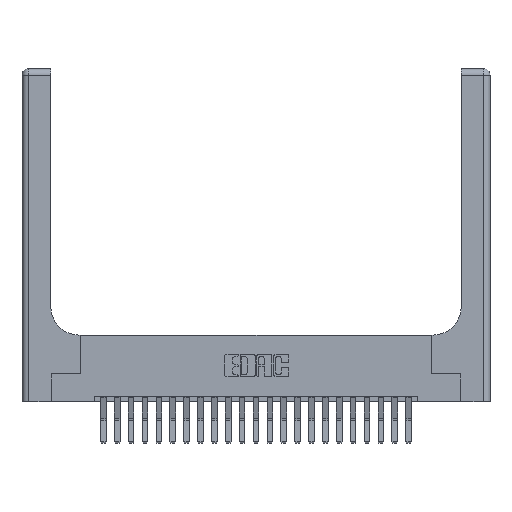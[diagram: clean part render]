
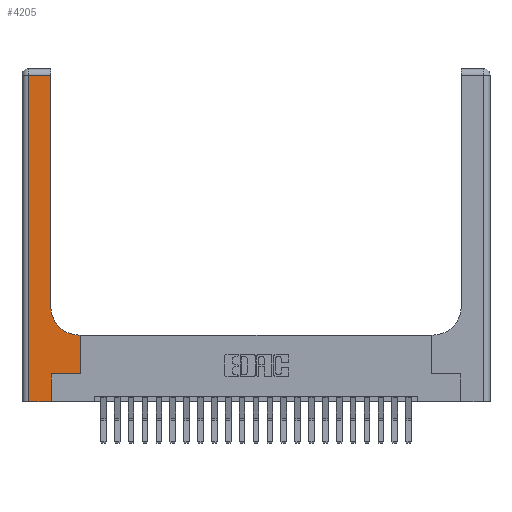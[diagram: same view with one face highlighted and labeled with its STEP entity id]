
A CAD part, top view. The second image highlights one B-rep face of the part: STEP entity #4205.
In plain terms, the highlighted planar face has unit normal (0, 0, 1).
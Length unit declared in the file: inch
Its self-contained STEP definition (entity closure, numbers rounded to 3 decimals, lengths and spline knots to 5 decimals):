
#377 = AXIS2_PLACEMENT_3D ( 'NONE', #8350, #18602, #2459 ) ;
#478 = DIRECTION ( 'NONE',  ( 0., 1., 0. ) ) ;
#1407 = LINE ( 'NONE', #3636, #17506 ) ;
#1566 = CARTESIAN_POINT ( 'NONE',  ( 0.06, 2.94, 0.37 ) ) ;
#1689 = CARTESIAN_POINT ( 'NONE',  ( 0.265, 0., 0.37 ) ) ;
#1898 = CARTESIAN_POINT ( 'NONE',  ( 0.528, 0.6, 0.37 ) ) ;
#2303 = ORIENTED_EDGE ( 'NONE', *, *, #22481, .T. ) ;
#2459 = DIRECTION ( 'NONE',  ( -1., 0., 0. ) ) ;
#2951 = LINE ( 'NONE', #11994, #8529 ) ;
#3006 = CARTESIAN_POINT ( 'NONE',  ( 0.06, 3., 0.37 ) ) ;
#3067 = DIRECTION ( 'NONE',  ( -1., 0., 0. ) ) ;
#3284 = VECTOR ( 'NONE', #478, 39.37008 ) ;
#3420 = LINE ( 'NONE', #19445, #11660 ) ;
#3590 = LINE ( 'NONE', #5131, #19628 ) ;
#3636 = CARTESIAN_POINT ( 'NONE',  ( 0., 0., 0.37 ) ) ;
#3974 = EDGE_CURVE ( 'NONE', #14510, #15277, #3420, .T. ) ;
#4205 = ADVANCED_FACE ( 'NONE', ( #11515 ), #10104, .F. ) ;
#4859 = EDGE_CURVE ( 'NONE', #9896, #6641, #21275, .T. ) ;
#4915 = ORIENTED_EDGE ( 'NONE', *, *, #15851, .T. ) ;
#5131 = CARTESIAN_POINT ( 'NONE',  ( 0., 2.94, 0.37 ) ) ;
#5249 = ORIENTED_EDGE ( 'NONE', *, *, #17344, .T. ) ;
#5640 = VECTOR ( 'NONE', #19911, 39.37008 ) ;
#6519 = LINE ( 'NONE', #3006, #11659 ) ;
#6641 = VERTEX_POINT ( 'NONE', #19539 ) ;
#6956 = CARTESIAN_POINT ( 'NONE',  ( 0.26, 2.94, 0.37 ) ) ;
#7289 = EDGE_CURVE ( 'NONE', #13634, #18597, #6519, .T. ) ;
#7962 = VERTEX_POINT ( 'NONE', #12374 ) ;
#8350 = CARTESIAN_POINT ( 'NONE',  ( 0., 3., 0.37 ) ) ;
#8529 = VECTOR ( 'NONE', #3067, 39.37008 ) ;
#8644 = DIRECTION ( 'NONE',  ( 0., -1., 0. ) ) ;
#9006 = DIRECTION ( 'NONE',  ( -1., 0., 0. ) ) ;
#9186 = ORIENTED_EDGE ( 'NONE', *, *, #17276, .T. ) ;
#9896 = VERTEX_POINT ( 'NONE', #1689 ) ;
#10104 = PLANE ( 'NONE',  #377 ) ;
#10374 = VERTEX_POINT ( 'NONE', #6956 ) ;
#10806 = DIRECTION ( 'NONE',  ( 1., 0., 0. ) ) ;
#11515 = FACE_OUTER_BOUND ( 'NONE', #15474, .T. ) ;
#11639 = ORIENTED_EDGE ( 'NONE', *, *, #7289, .T. ) ;
#11660 = VECTOR ( 'NONE', #21550, 39.37008 ) ;
#11659 = VECTOR ( 'NONE', #8644, 39.37008 ) ;
#11994 = CARTESIAN_POINT ( 'NONE',  ( 0.26, 0.6, 0.37 ) ) ;
#12073 = EDGE_CURVE ( 'NONE', #7962, #10374, #21552, .T. ) ;
#12080 = DIRECTION ( 'NONE',  ( 0., 0., -1. ) ) ;
#12310 = DIRECTION ( 'NONE',  ( 1., 0., 0. ) ) ;
#12374 = CARTESIAN_POINT ( 'NONE',  ( 0.26, 0.85, 0.37 ) ) ;
#12739 = CIRCLE ( 'NONE', #17637, 0.25 ) ;
#13257 = VERTEX_POINT ( 'NONE', #20452 ) ;
#13634 = VERTEX_POINT ( 'NONE', #1566 ) ;
#14020 = ORIENTED_EDGE ( 'NONE', *, *, #12073, .T. ) ;
#14229 = CARTESIAN_POINT ( 'NONE',  ( 0.265, 0.25, 0.37 ) ) ;
#14510 = VERTEX_POINT ( 'NONE', #20108 ) ;
#14983 = VECTOR ( 'NONE', #21436, 39.37008 ) ;
#15277 = VERTEX_POINT ( 'NONE', #1898 ) ;
#15474 = EDGE_LOOP ( 'NONE', ( #14020, #5249, #11639, #17322, #16744, #4915, #17448, #2303, #9186 ) ) ;
#15787 = EDGE_CURVE ( 'NONE', #18597, #9896, #1407, .T. ) ;
#15851 = EDGE_CURVE ( 'NONE', #6641, #14510, #23199, .T. ) ;
#16229 = CARTESIAN_POINT ( 'NONE',  ( 0.26, 3., 0.37 ) ) ;
#16744 = ORIENTED_EDGE ( 'NONE', *, *, #4859, .T. ) ;
#16800 = CARTESIAN_POINT ( 'NONE',  ( 0.06, 0., 0.37 ) ) ;
#17276 = EDGE_CURVE ( 'NONE', #13257, #7962, #12739, .T. ) ;
#17322 = ORIENTED_EDGE ( 'NONE', *, *, #15787, .T. ) ;
#17344 = EDGE_CURVE ( 'NONE', #10374, #13634, #3590, .T. ) ;
#17448 = ORIENTED_EDGE ( 'NONE', *, *, #3974, .T. ) ;
#17506 = VECTOR ( 'NONE', #10806, 39.37008 ) ;
#17637 = AXIS2_PLACEMENT_3D ( 'NONE', #23152, #12080, #12310 ) ;
#18597 = VERTEX_POINT ( 'NONE', #16800 ) ;
#18602 = DIRECTION ( 'NONE',  ( 0., 0., -1. ) ) ;
#19445 = CARTESIAN_POINT ( 'NONE',  ( 0.528, 0.25, 0.37 ) ) ;
#19539 = CARTESIAN_POINT ( 'NONE',  ( 0.265, 0.25, 0.37 ) ) ;
#19628 = VECTOR ( 'NONE', #9006, 39.37008 ) ;
#19911 = DIRECTION ( 'NONE',  ( 0., 1., 0. ) ) ;
#20108 = CARTESIAN_POINT ( 'NONE',  ( 0.528, 0.25, 0.37 ) ) ;
#20170 = CARTESIAN_POINT ( 'NONE',  ( 0.265, 0., 0.37 ) ) ;
#20452 = CARTESIAN_POINT ( 'NONE',  ( 0.51, 0.6, 0.37 ) ) ;
#21275 = LINE ( 'NONE', #20170, #3284 ) ;
#21436 = DIRECTION ( 'NONE',  ( 1., 0., 0. ) ) ;
#21550 = DIRECTION ( 'NONE',  ( 0., 1., 0. ) ) ;
#21552 = LINE ( 'NONE', #16229, #5640 ) ;
#22481 = EDGE_CURVE ( 'NONE', #15277, #13257, #2951, .T. ) ;
#23152 = CARTESIAN_POINT ( 'NONE',  ( 0.51, 0.85, 0.37 ) ) ;
#23199 = LINE ( 'NONE', #14229, #14983 ) ;
